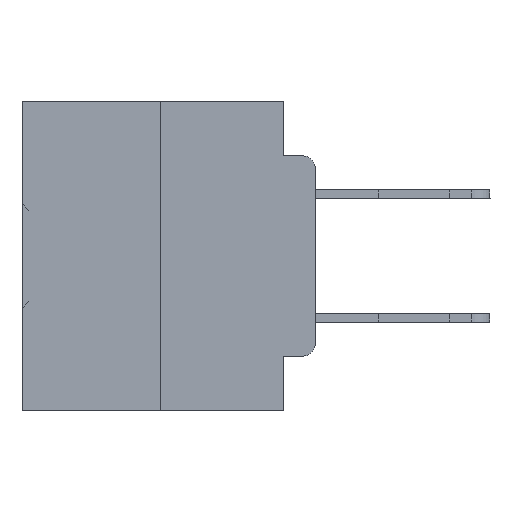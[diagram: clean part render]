
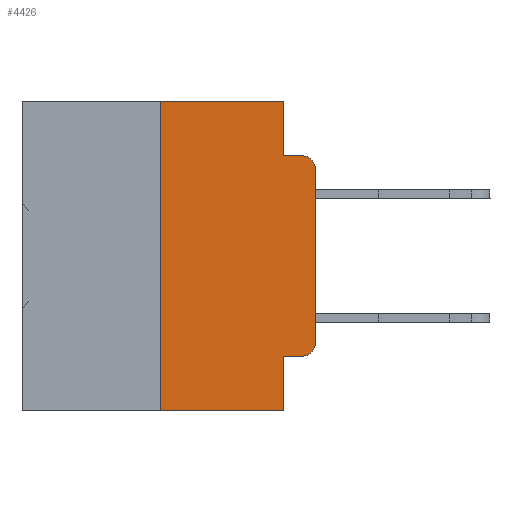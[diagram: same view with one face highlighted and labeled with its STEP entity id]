
A CAD part, left-side view. The second image highlights one B-rep face of the part: STEP entity #4426.
In plain terms, the highlighted planar face has unit normal (-1, 0, 0).
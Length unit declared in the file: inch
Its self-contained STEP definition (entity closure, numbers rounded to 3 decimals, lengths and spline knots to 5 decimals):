
#163 = DIRECTION ( 'NONE',  ( -1., 0., 0. ) ) ;
#610 = EDGE_CURVE ( 'NONE', #33227, #32631, #37141, .T. ) ;
#1076 = VECTOR ( 'NONE', #1085, 39.37008 ) ;
#1085 = DIRECTION ( 'NONE',  ( 0., -1., 0. ) ) ;
#2267 = FACE_OUTER_BOUND ( 'NONE', #25347, .T. ) ;
#2374 = EDGE_CURVE ( 'NONE', #25138, #10751, #30315, .T. ) ;
#2574 = EDGE_CURVE ( 'NONE', #19417, #32631, #28993, .T. ) ;
#3071 = ORIENTED_EDGE ( 'NONE', *, *, #18687, .T. ) ;
#3648 = CARTESIAN_POINT ( 'NONE',  ( 0., 0.051, -0.4115 ) ) ;
#3729 = VECTOR ( 'NONE', #34736, 39.37008 ) ;
#3936 = CARTESIAN_POINT ( 'NONE',  ( 0., 0.051, 0. ) ) ;
#4426 = ADVANCED_FACE ( 'NONE', ( #2267 ), #14790, .F. ) ;
#4615 = VECTOR ( 'NONE', #9417, 39.37008 ) ;
#5180 = CARTESIAN_POINT ( 'NONE',  ( 0., 0., -0.3915 ) ) ;
#5652 = ORIENTED_EDGE ( 'NONE', *, *, #17042, .T. ) ;
#6626 = VECTOR ( 'NONE', #37727, 39.37008 ) ;
#6995 = VERTEX_POINT ( 'NONE', #27532 ) ;
#7211 = DIRECTION ( 'NONE',  ( 0., -1., 0. ) ) ;
#9314 = DIRECTION ( 'NONE',  ( 0., 0., -1. ) ) ;
#9417 = DIRECTION ( 'NONE',  ( 0., 0., -1. ) ) ;
#9696 = CARTESIAN_POINT ( 'NONE',  ( 0., 0.473, -0.5 ) ) ;
#10286 = VECTOR ( 'NONE', #26353, 39.37008 ) ;
#10355 = EDGE_CURVE ( 'NONE', #16359, #22284, #21294, .T. ) ;
#10751 = VERTEX_POINT ( 'NONE', #5180 ) ;
#12292 = CARTESIAN_POINT ( 'NONE',  ( 0., 0.02, -0.0885 ) ) ;
#13153 = AXIS2_PLACEMENT_3D ( 'NONE', #24249, #163, #9314 ) ;
#13486 = DIRECTION ( 'NONE',  ( 0., -1., 0. ) ) ;
#14790 = PLANE ( 'NONE',  #19624 ) ;
#15373 = CARTESIAN_POINT ( 'NONE',  ( 0., 0.051, 0. ) ) ;
#15463 = CARTESIAN_POINT ( 'NONE',  ( 0., 0., -0.1085 ) ) ;
#16161 = LINE ( 'NONE', #3648, #39001 ) ;
#16196 = LINE ( 'NONE', #37868, #1076 ) ;
#16359 = VERTEX_POINT ( 'NONE', #15463 ) ;
#16567 = DIRECTION ( 'NONE',  ( -1., 0., 0. ) ) ;
#16847 = ORIENTED_EDGE ( 'NONE', *, *, #23690, .F. ) ;
#16933 = VERTEX_POINT ( 'NONE', #37494 ) ;
#17042 = EDGE_CURVE ( 'NONE', #10751, #16359, #23166, .T. ) ;
#17321 = EDGE_CURVE ( 'NONE', #16933, #33106, #33700, .T. ) ;
#18261 = ORIENTED_EDGE ( 'NONE', *, *, #2574, .F. ) ;
#18687 = EDGE_CURVE ( 'NONE', #19417, #25138, #16161, .T. ) ;
#18823 = LINE ( 'NONE', #34530, #3729 ) ;
#19069 = LINE ( 'NONE', #19252, #37256 ) ;
#19252 = CARTESIAN_POINT ( 'NONE',  ( 0., 0.051, -0.0885 ) ) ;
#19417 = VERTEX_POINT ( 'NONE', #38502 ) ;
#19624 = AXIS2_PLACEMENT_3D ( 'NONE', #26941, #26355, #32118 ) ;
#21294 = CIRCLE ( 'NONE', #39087, 0.02 ) ;
#22284 = VERTEX_POINT ( 'NONE', #12292 ) ;
#22626 = ORIENTED_EDGE ( 'NONE', *, *, #36646, .F. ) ;
#23166 = LINE ( 'NONE', #25964, #10286 ) ;
#23690 = EDGE_CURVE ( 'NONE', #33106, #22284, #19069, .T. ) ;
#24249 = CARTESIAN_POINT ( 'NONE',  ( 0., 0.02, -0.3915 ) ) ;
#25138 = VERTEX_POINT ( 'NONE', #32384 ) ;
#25347 = EDGE_LOOP ( 'NONE', ( #5652, #32492, #16847, #25475, #22626, #28879, #34337, #18261, #3071, #30127 ) ) ;
#25475 = ORIENTED_EDGE ( 'NONE', *, *, #17321, .F. ) ;
#25540 = EDGE_CURVE ( 'NONE', #33227, #6995, #18823, .T. ) ;
#25964 = CARTESIAN_POINT ( 'NONE',  ( 0., 0., 0. ) ) ;
#26353 = DIRECTION ( 'NONE',  ( 0., 0., 1. ) ) ;
#26355 = DIRECTION ( 'NONE',  ( 1., 0., 0. ) ) ;
#26673 = CARTESIAN_POINT ( 'NONE',  ( 0., 0.051, -0.0885 ) ) ;
#26941 = CARTESIAN_POINT ( 'NONE',  ( 0., 0.473, 0. ) ) ;
#27532 = CARTESIAN_POINT ( 'NONE',  ( 0., 0.25, 0. ) ) ;
#28208 = DIRECTION ( 'NONE',  ( 0., 0., -1. ) ) ;
#28879 = ORIENTED_EDGE ( 'NONE', *, *, #25540, .F. ) ;
#28993 = LINE ( 'NONE', #3936, #34774 ) ;
#30127 = ORIENTED_EDGE ( 'NONE', *, *, #2374, .T. ) ;
#30315 = CIRCLE ( 'NONE', #13153, 0.02 ) ;
#32118 = DIRECTION ( 'NONE',  ( 0., 0., -1. ) ) ;
#32384 = CARTESIAN_POINT ( 'NONE',  ( 0., 0.02, -0.4115 ) ) ;
#32492 = ORIENTED_EDGE ( 'NONE', *, *, #10355, .T. ) ;
#32631 = VERTEX_POINT ( 'NONE', #35317 ) ;
#33106 = VERTEX_POINT ( 'NONE', #26673 ) ;
#33227 = VERTEX_POINT ( 'NONE', #36403 ) ;
#33700 = LINE ( 'NONE', #15373, #4615 ) ;
#34337 = ORIENTED_EDGE ( 'NONE', *, *, #610, .T. ) ;
#34530 = CARTESIAN_POINT ( 'NONE',  ( 0., 0.25, 0. ) ) ;
#34736 = DIRECTION ( 'NONE',  ( 0., 0., 1. ) ) ;
#34774 = VECTOR ( 'NONE', #28208, 39.37008 ) ;
#35078 = DIRECTION ( 'NONE',  ( 0., 0., -1. ) ) ;
#35317 = CARTESIAN_POINT ( 'NONE',  ( 0., 0.051, -0.5 ) ) ;
#36403 = CARTESIAN_POINT ( 'NONE',  ( 0., 0.25, -0.5 ) ) ;
#36646 = EDGE_CURVE ( 'NONE', #6995, #16933, #16196, .T. ) ;
#37141 = LINE ( 'NONE', #9696, #6626 ) ;
#37256 = VECTOR ( 'NONE', #13486, 39.37008 ) ;
#37494 = CARTESIAN_POINT ( 'NONE',  ( 0., 0.051, 0. ) ) ;
#37727 = DIRECTION ( 'NONE',  ( 0., -1., 0. ) ) ;
#37868 = CARTESIAN_POINT ( 'NONE',  ( 0., 0.473, 0. ) ) ;
#38441 = CARTESIAN_POINT ( 'NONE',  ( 0., 0.02, -0.1085 ) ) ;
#38502 = CARTESIAN_POINT ( 'NONE',  ( 0., 0.051, -0.4115 ) ) ;
#39001 = VECTOR ( 'NONE', #7211, 39.37008 ) ;
#39087 = AXIS2_PLACEMENT_3D ( 'NONE', #38441, #16567, #35078 ) ;
